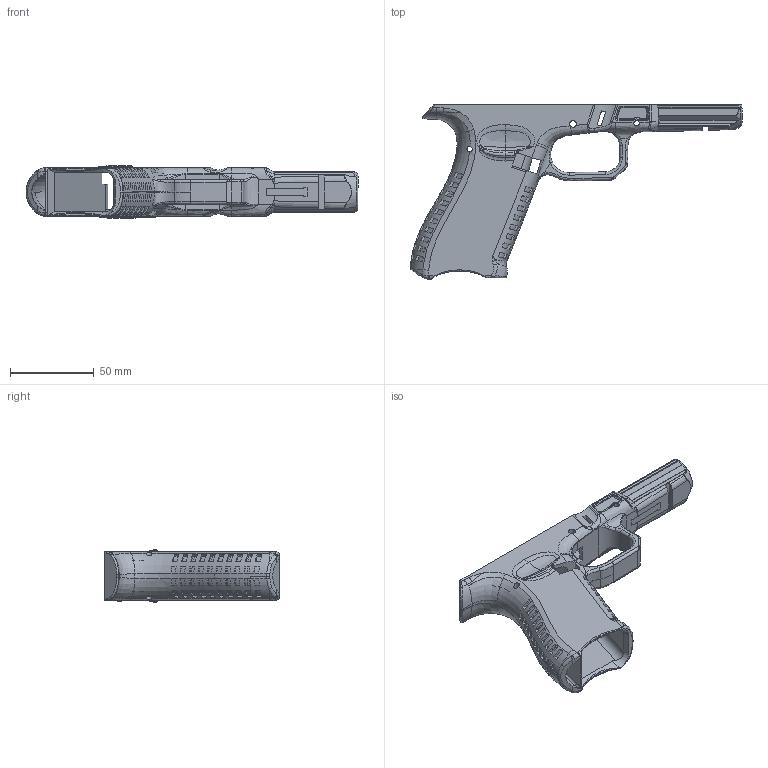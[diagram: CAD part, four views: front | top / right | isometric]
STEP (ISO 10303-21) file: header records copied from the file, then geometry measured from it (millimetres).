
FILE_DESCRIPTION(/* description */ (''),/* implementation_level */ '2;1');
FILE_NAME(/* name */ 'PY2A G17 Frame (FFFTech Mod).step',/* time_stamp */ '2021-02-25T02:11:25-05:00',/* author */ (''),/* organization */ (''),/* preprocessor_version */ 'ST-DEVELOPER v18.1',/* originating_system */ 'Autodesk Translation Framework v9.7.1.1290',/* authorisation */ '');
FILE_SCHEMA (('AUTOMOTIVE_DESIGN { 1 0 10303 214 3 1 1 }'));
Products named in the file (1): PrintYour2A G17 Frame (FFFTech Mod)
Bounding box: 197.76 x 104 x 31.4 mm (x, y, z)
Volume: 80907 mm3; surface area: 52437.4 mm2
Topology: 1 solids, 1 shells, 1212 faces, 3255 edges, 2065 vertices
Faces by surface type: bspline 541, plane 496, cylinder 141, torus 19, sphere 10, cone 5
Full cylindrical faces by diameter (mm): 1.5 x2, 3.225 x2, 3.25 x2, 4.05 x2
Entity records: 107350 total; most frequent: CARTESIAN_POINT 80902, ORIENTED_EDGE 6470, DIRECTION 3994, EDGE_CURVE 3235, VERTEX_POINT 2065, AXIS2_PLACEMENT_3D 1386, B_SPLINE_CURVE_WITH_KNOTS 1296, EDGE_LOOP 1278
